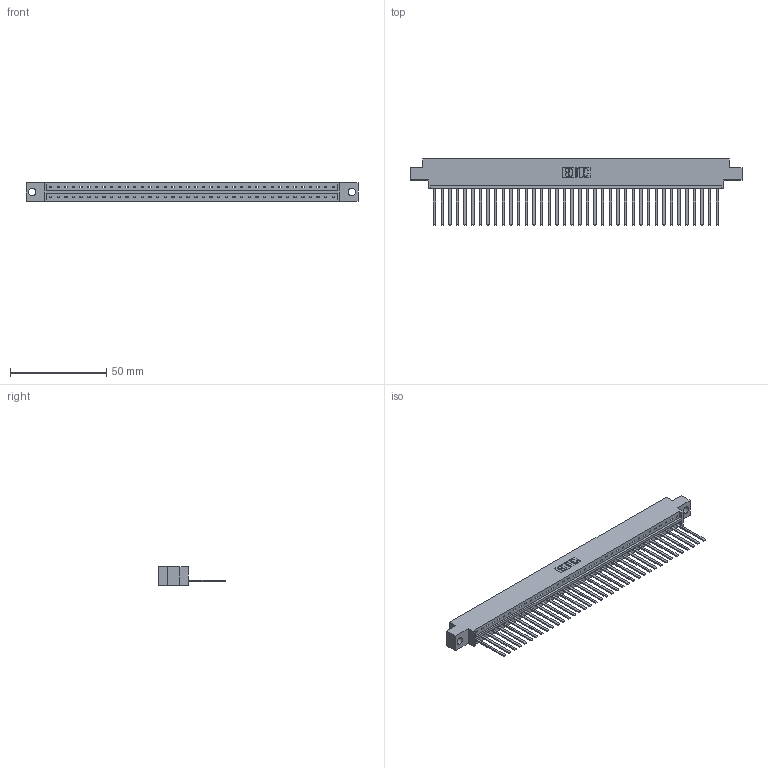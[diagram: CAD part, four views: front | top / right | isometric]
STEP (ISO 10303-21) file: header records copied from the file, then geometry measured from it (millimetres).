
FILE_DESCRIPTION (( 'STEP AP203' ), '1' );
FILE_NAME ('833-038-544-604.STEP', '2020-06-03T13:16:30', ( '' ), ( '' ), 'SwSTEP 2.0', 'SolidWorks 2020', '' );
FILE_SCHEMA (( 'CONFIG_CONTROL_DESIGN' ));
Length unit declared in the file: inch
Products named in the file (3): 833 Part_Offset - .156 Dia - TH; 833-038-544-604; 345-292-001_345-293-144
Assembly tree (39 placements, depth 2):
  833-038-544-604
    833 Part_Offset - .156 Dia - TH
    345-292-001_345-293-144  x38
Bounding box: 172.11 x 34.3 x 9.4 mm (x, y, z)
Volume: 17409.2 mm3; surface area: 20234.7 mm2
Topology: 39 solids, 39 shells, 2094 faces, 6327 edges, 4166 vertices
Faces by surface type: plane 1518, cylinder 576
Entity records: 23699 total; most frequent: CARTESIAN_POINT 4096, ORIENTED_EDGE 4070, DIRECTION 3459, EDGE_CURVE 2035, VECTOR 1911, LINE 1911, VERTEX_POINT 1354, AXIS2_PLACEMENT_3D 774
